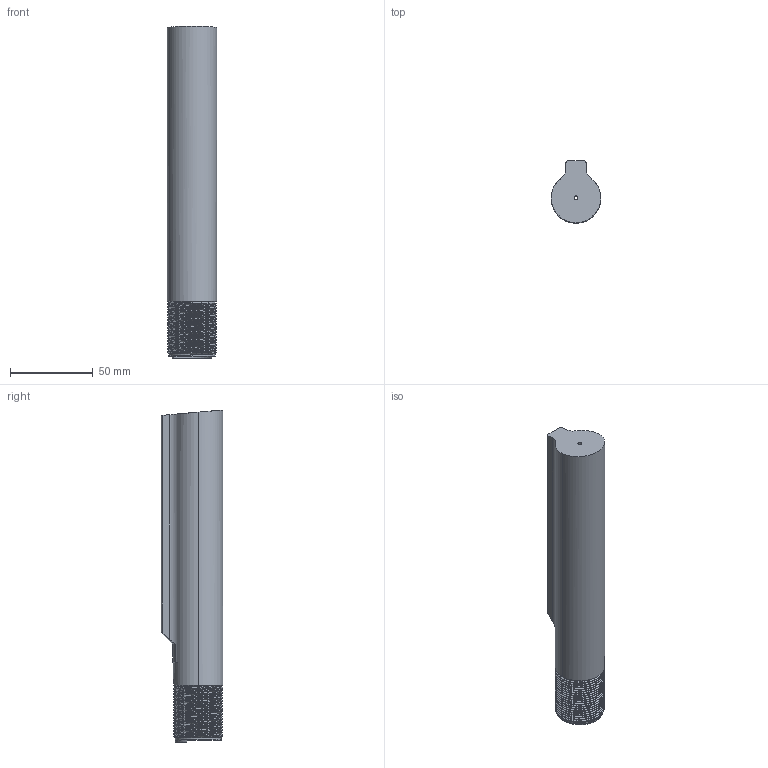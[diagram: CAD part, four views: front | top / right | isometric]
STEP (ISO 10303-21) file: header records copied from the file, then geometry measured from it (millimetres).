
FILE_DESCRIPTION (( 'STEP AP214' ), '1' );
FILE_NAME ('User Library-Telescopic Stock_Telescopic Stock Tube1.STEP', '2013-05-23T12:55:35', ( 'Asher' ), ( '' ), 'SwSTEP 2.0', 'SolidWorks 2013', '' );
FILE_SCHEMA (( 'AUTOMOTIVE_DESIGN' ));
Length unit declared in the file: millimetre
Products named in the file (1): User Library-Telescopic Stock_Telescopic Stock Tube1
Bounding box: 29.84 x 37.34 x 200.02 mm (x, y, z)
Volume: 55765.2 mm3; surface area: 39989.2 mm2
Topology: 1 solids, 1 shells, 224 faces, 638 edges, 421 vertices
Faces by surface type: cylinder 109, plane 62, bspline 42, cone 11
Entity records: 16642 total; most frequent: CARTESIAN_POINT 11875, ORIENTED_EDGE 1276, DIRECTION 673, EDGE_CURVE 638, VERTEX_POINT 421, AXIS2_PLACEMENT_3D 248, EDGE_LOOP 231, ADVANCED_FACE 224
